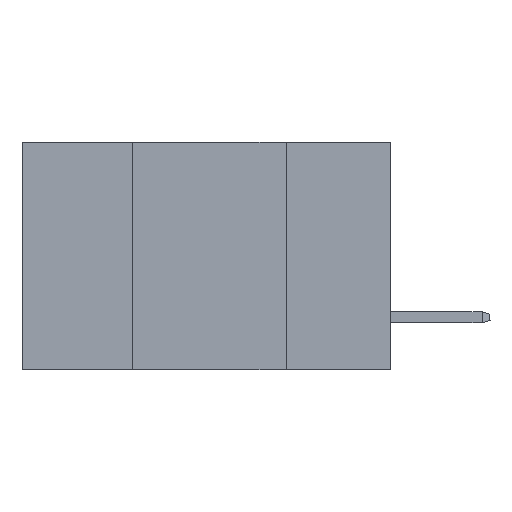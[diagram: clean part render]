
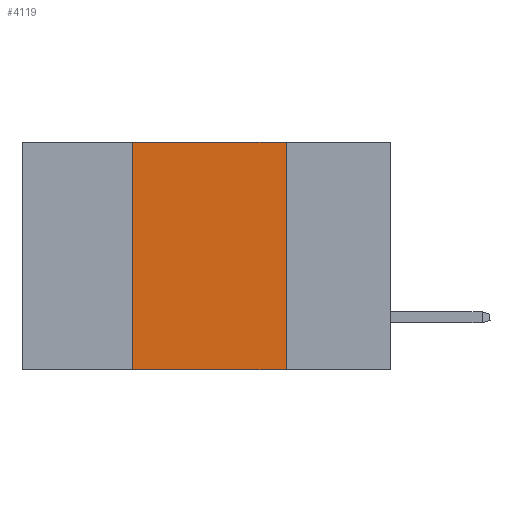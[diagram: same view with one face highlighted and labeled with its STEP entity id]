
A CAD part, left-side view. The second image highlights one B-rep face of the part: STEP entity #4119.
In plain terms, the highlighted planar face has unit normal (-1, 0, 0).
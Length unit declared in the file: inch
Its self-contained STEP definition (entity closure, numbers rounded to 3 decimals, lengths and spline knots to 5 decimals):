
#931 = AXIS2_PLACEMENT_3D ( 'NONE', #17936, #20299, #5565 ) ;
#997 = CARTESIAN_POINT ( 'NONE',  ( 0., 0.6, 0. ) ) ;
#1825 = CARTESIAN_POINT ( 'NONE',  ( 0., 0.17, 0. ) ) ;
#2909 = CARTESIAN_POINT ( 'NONE',  ( 0., 0.17, 0. ) ) ;
#3601 = VECTOR ( 'NONE', #8077, 39.37008 ) ;
#3603 = EDGE_CURVE ( 'NONE', #24808, #6826, #9180, .T. ) ;
#4119 = ADVANCED_FACE ( 'NONE', ( #22592 ), #9593, .F. ) ;
#5413 = ORIENTED_EDGE ( 'NONE', *, *, #6622, .T. ) ;
#5565 = DIRECTION ( 'NONE',  ( 0., 0., -1. ) ) ;
#6453 = LINE ( 'NONE', #10558, #15934 ) ;
#6622 = EDGE_CURVE ( 'NONE', #13283, #6826, #20791, .T. ) ;
#6826 = VERTEX_POINT ( 'NONE', #22463 ) ;
#8077 = DIRECTION ( 'NONE',  ( 0., 0., -1. ) ) ;
#9180 = LINE ( 'NONE', #1825, #3601 ) ;
#9593 = PLANE ( 'NONE',  #931 ) ;
#10558 = CARTESIAN_POINT ( 'NONE',  ( 0., 0.42, 0. ) ) ;
#11543 = EDGE_LOOP ( 'NONE', ( #16851, #18430, #23537, #5413 ) ) ;
#12263 = CARTESIAN_POINT ( 'NONE',  ( 0., 0.42, 0. ) ) ;
#12331 = EDGE_CURVE ( 'NONE', #13283, #24513, #6453, .T. ) ;
#12456 = VECTOR ( 'NONE', #25996, 39.37008 ) ;
#13283 = VERTEX_POINT ( 'NONE', #22721 ) ;
#15934 = VECTOR ( 'NONE', #16672, 39.37008 ) ;
#16672 = DIRECTION ( 'NONE',  ( 0., 0., 1. ) ) ;
#16851 = ORIENTED_EDGE ( 'NONE', *, *, #3603, .F. ) ;
#17936 = CARTESIAN_POINT ( 'NONE',  ( 0., 0.6, 0. ) ) ;
#18430 = ORIENTED_EDGE ( 'NONE', *, *, #25412, .F. ) ;
#20299 = DIRECTION ( 'NONE',  ( 1., 0., 0. ) ) ;
#20791 = LINE ( 'NONE', #21154, #21439 ) ;
#21154 = CARTESIAN_POINT ( 'NONE',  ( 0., 0.6, -0.37 ) ) ;
#21439 = VECTOR ( 'NONE', #23527, 39.37008 ) ;
#22463 = CARTESIAN_POINT ( 'NONE',  ( 0., 0.17, -0.37 ) ) ;
#22592 = FACE_OUTER_BOUND ( 'NONE', #11543, .T. ) ;
#22721 = CARTESIAN_POINT ( 'NONE',  ( 0., 0.42, -0.37 ) ) ;
#23527 = DIRECTION ( 'NONE',  ( 0., -1., 0. ) ) ;
#23537 = ORIENTED_EDGE ( 'NONE', *, *, #12331, .F. ) ;
#24513 = VERTEX_POINT ( 'NONE', #12263 ) ;
#24808 = VERTEX_POINT ( 'NONE', #2909 ) ;
#25088 = LINE ( 'NONE', #997, #12456 ) ;
#25412 = EDGE_CURVE ( 'NONE', #24513, #24808, #25088, .T. ) ;
#25996 = DIRECTION ( 'NONE',  ( 0., -1., 0. ) ) ;
